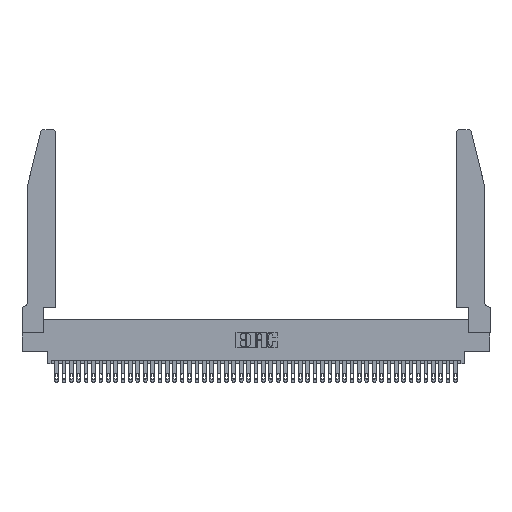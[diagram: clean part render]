
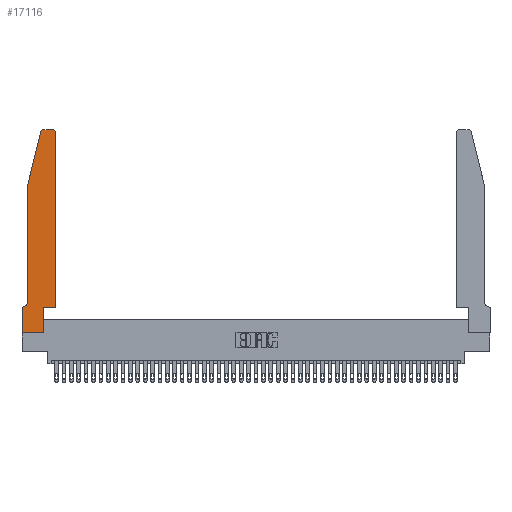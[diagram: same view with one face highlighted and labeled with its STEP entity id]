
A CAD part, top view. The second image highlights one B-rep face of the part: STEP entity #17116.
In plain terms, the highlighted planar face has unit normal (0, 0, 1).
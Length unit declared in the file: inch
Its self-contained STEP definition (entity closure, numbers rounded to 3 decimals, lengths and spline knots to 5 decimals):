
#205 = VERTEX_POINT ( 'NONE', #23866 ) ;
#243 = EDGE_CURVE ( 'NONE', #15219, #40441, #8505, .T. ) ;
#551 = AXIS2_PLACEMENT_3D ( 'NONE', #6608, #21176, #28398 ) ;
#1080 = CARTESIAN_POINT ( 'NONE',  ( 0.2605, 2.75, 0.37 ) ) ;
#2054 = LINE ( 'NONE', #35041, #45600 ) ;
#2274 = ORIENTED_EDGE ( 'NONE', *, *, #34450, .T. ) ;
#2514 = CARTESIAN_POINT ( 'NONE',  ( 0.284, 2.72, 0.37 ) ) ;
#2530 = CARTESIAN_POINT ( 'NONE',  ( 0.4205, 2.75, 0.37 ) ) ;
#2793 = CARTESIAN_POINT ( 'NONE',  ( 0.2865, 0.35, 0.37 ) ) ;
#3098 = CIRCLE ( 'NONE', #551, 0.03 ) ;
#3271 = EDGE_CURVE ( 'NONE', #205, #31081, #39086, .T. ) ;
#3389 = VERTEX_POINT ( 'NONE', #41378 ) ;
#3794 = ORIENTED_EDGE ( 'NONE', *, *, #22959, .T. ) ;
#4075 = CARTESIAN_POINT ( 'NONE',  ( 0., 0.35, 0.37 ) ) ;
#4686 = DIRECTION ( 'NONE',  ( -1., 0., 0. ) ) ;
#5202 = CARTESIAN_POINT ( 'NONE',  ( 0.4505, 0.35, 0.37 ) ) ;
#5701 = CARTESIAN_POINT ( 'NONE',  ( 0., 0.35, 0.37 ) ) ;
#6179 = CARTESIAN_POINT ( 'NONE',  ( 0.0755, 0.35, 0.37 ) ) ;
#6476 = ORIENTED_EDGE ( 'NONE', *, *, #24324, .T. ) ;
#6608 = CARTESIAN_POINT ( 'NONE',  ( 0.4205, 2.72, 0.37 ) ) ;
#7022 = CARTESIAN_POINT ( 'NONE',  ( 0.0755, 2., 0.37 ) ) ;
#7661 = DIRECTION ( 'NONE',  ( -1., 0., 0. ) ) ;
#7772 = EDGE_LOOP ( 'NONE', ( #2274, #37544, #17018, #6476, #20443, #32342, #44860, #3794, #15567, #26046, #33682, #15387 ) ) ;
#7820 = LINE ( 'NONE', #1080, #19067 ) ;
#8293 = CARTESIAN_POINT ( 'NONE',  ( 0.2865, 0., 0.37 ) ) ;
#8505 = LINE ( 'NONE', #10660, #15821 ) ;
#8669 = CARTESIAN_POINT ( 'NONE',  ( 0.4505, 2.72, 0.37 ) ) ;
#9357 = EDGE_CURVE ( 'NONE', #31081, #35179, #2054, .T. ) ;
#9649 = DIRECTION ( 'NONE',  ( -1., 0., 0. ) ) ;
#10660 = CARTESIAN_POINT ( 'NONE',  ( 0.4505, 0.35, 0.37 ) ) ;
#11590 = VECTOR ( 'NONE', #15025, 39.37008 ) ;
#11599 = CARTESIAN_POINT ( 'NONE',  ( 0.0055, 0.42, 0.37 ) ) ;
#12109 = EDGE_CURVE ( 'NONE', #14781, #20283, #23938, .T. ) ;
#13321 = CARTESIAN_POINT ( 'NONE',  ( 0.25487, 2.72718, 0.37 ) ) ;
#13514 = VERTEX_POINT ( 'NONE', #16440 ) ;
#13617 = LINE ( 'NONE', #2793, #21993 ) ;
#13639 = LINE ( 'NONE', #7022, #14238 ) ;
#13769 = AXIS2_PLACEMENT_3D ( 'NONE', #5701, #44553, #26834 ) ;
#14238 = VECTOR ( 'NONE', #28814, 39.37008 ) ;
#14781 = VERTEX_POINT ( 'NONE', #4075 ) ;
#15025 = DIRECTION ( 'NONE',  ( 0., -1., 0. ) ) ;
#15219 = VERTEX_POINT ( 'NONE', #17359 ) ;
#15387 = ORIENTED_EDGE ( 'NONE', *, *, #29492, .T. ) ;
#15567 = ORIENTED_EDGE ( 'NONE', *, *, #45904, .T. ) ;
#15821 = VECTOR ( 'NONE', #42945, 39.37008 ) ;
#16440 = CARTESIAN_POINT ( 'NONE',  ( 0.0755, 0.42, 0.37 ) ) ;
#17018 = ORIENTED_EDGE ( 'NONE', *, *, #9357, .T. ) ;
#17116 = ADVANCED_FACE ( 'NONE', ( #39801 ), #30467, .T. ) ;
#17359 = CARTESIAN_POINT ( 'NONE',  ( 0.2865, 0.35, 0.37 ) ) ;
#17582 = VERTEX_POINT ( 'NONE', #2530 ) ;
#19067 = VECTOR ( 'NONE', #4686, 39.37008 ) ;
#19277 = CIRCLE ( 'NONE', #40746, 0.07 ) ;
#19767 = EDGE_CURVE ( 'NONE', #13514, #3389, #19277, .T. ) ;
#20281 = CARTESIAN_POINT ( 'NONE',  ( 0.0755, 2., 0.37 ) ) ;
#20283 = VERTEX_POINT ( 'NONE', #31448 ) ;
#20443 = ORIENTED_EDGE ( 'NONE', *, *, #19767, .T. ) ;
#20511 = DIRECTION ( 'NONE',  ( 0., 1., 0. ) ) ;
#20875 = LINE ( 'NONE', #5202, #39853 ) ;
#21176 = DIRECTION ( 'NONE',  ( 0., 0., 1. ) ) ;
#21993 = VECTOR ( 'NONE', #38565, 39.37008 ) ;
#22469 = LINE ( 'NONE', #43723, #29781 ) ;
#22564 = DIRECTION ( 'NONE',  ( 0., 0., -1. ) ) ;
#22959 = EDGE_CURVE ( 'NONE', #20283, #25845, #22469, .T. ) ;
#23093 = AXIS2_PLACEMENT_3D ( 'NONE', #2514, #27556, #31150 ) ;
#23848 = EDGE_CURVE ( 'NONE', #3389, #14781, #30456, .T. ) ;
#23866 = CARTESIAN_POINT ( 'NONE',  ( 0.284, 2.75, 0.37 ) ) ;
#23938 = LINE ( 'NONE', #36253, #11590 ) ;
#24324 = EDGE_CURVE ( 'NONE', #35179, #13514, #13639, .T. ) ;
#25219 = VERTEX_POINT ( 'NONE', #8669 ) ;
#25845 = VERTEX_POINT ( 'NONE', #8293 ) ;
#26046 = ORIENTED_EDGE ( 'NONE', *, *, #243, .T. ) ;
#26834 = DIRECTION ( 'NONE',  ( 1., 0., 0. ) ) ;
#27556 = DIRECTION ( 'NONE',  ( 0., 0., 1. ) ) ;
#28398 = DIRECTION ( 'NONE',  ( 1., 0., 0. ) ) ;
#28814 = DIRECTION ( 'NONE',  ( 0., -1., 0. ) ) ;
#29492 = EDGE_CURVE ( 'NONE', #25219, #17582, #3098, .T. ) ;
#29781 = VECTOR ( 'NONE', #33823, 39.37008 ) ;
#30456 = LINE ( 'NONE', #6179, #34868 ) ;
#30467 = PLANE ( 'NONE',  #13769 ) ;
#31081 = VERTEX_POINT ( 'NONE', #13321 ) ;
#31150 = DIRECTION ( 'NONE',  ( 1., 0., 0. ) ) ;
#31448 = CARTESIAN_POINT ( 'NONE',  ( 0., 0., 0.37 ) ) ;
#32342 = ORIENTED_EDGE ( 'NONE', *, *, #23848, .T. ) ;
#33682 = ORIENTED_EDGE ( 'NONE', *, *, #40211, .T. ) ;
#33823 = DIRECTION ( 'NONE',  ( 1., 0., 0. ) ) ;
#34450 = EDGE_CURVE ( 'NONE', #17582, #205, #7820, .T. ) ;
#34868 = VECTOR ( 'NONE', #9649, 39.37008 ) ;
#35041 = CARTESIAN_POINT ( 'NONE',  ( 0.0755, 2., 0.37 ) ) ;
#35179 = VERTEX_POINT ( 'NONE', #20281 ) ;
#36253 = CARTESIAN_POINT ( 'NONE',  ( 0., 0., 0.37 ) ) ;
#37544 = ORIENTED_EDGE ( 'NONE', *, *, #3271, .T. ) ;
#38565 = DIRECTION ( 'NONE',  ( 0., 1., 0. ) ) ;
#38753 = DIRECTION ( 'NONE',  ( -0.239, -0.971, 0. ) ) ;
#39086 = CIRCLE ( 'NONE', #23093, 0.03 ) ;
#39801 = FACE_OUTER_BOUND ( 'NONE', #7772, .T. ) ;
#39853 = VECTOR ( 'NONE', #20511, 39.37008 ) ;
#40211 = EDGE_CURVE ( 'NONE', #40441, #25219, #20875, .T. ) ;
#40441 = VERTEX_POINT ( 'NONE', #42492 ) ;
#40746 = AXIS2_PLACEMENT_3D ( 'NONE', #11599, #22564, #7661 ) ;
#41378 = CARTESIAN_POINT ( 'NONE',  ( 0.0055, 0.35, 0.37 ) ) ;
#42492 = CARTESIAN_POINT ( 'NONE',  ( 0.4505, 0.35, 0.37 ) ) ;
#42945 = DIRECTION ( 'NONE',  ( 1., 0., 0. ) ) ;
#43723 = CARTESIAN_POINT ( 'NONE',  ( 0., 0., 0.37 ) ) ;
#44553 = DIRECTION ( 'NONE',  ( 0., 0., 1. ) ) ;
#44860 = ORIENTED_EDGE ( 'NONE', *, *, #12109, .T. ) ;
#45600 = VECTOR ( 'NONE', #38753, 39.37008 ) ;
#45904 = EDGE_CURVE ( 'NONE', #25845, #15219, #13617, .T. ) ;
